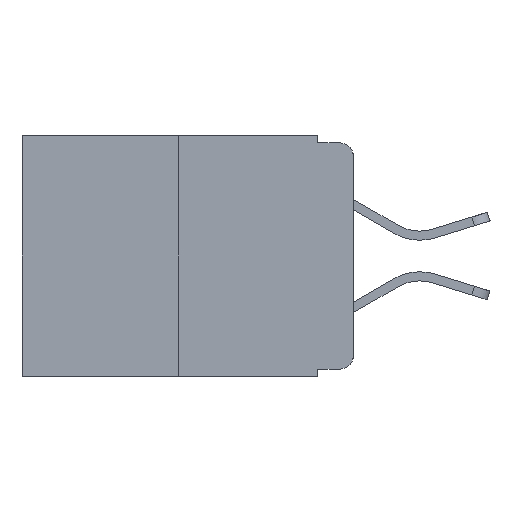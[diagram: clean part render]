
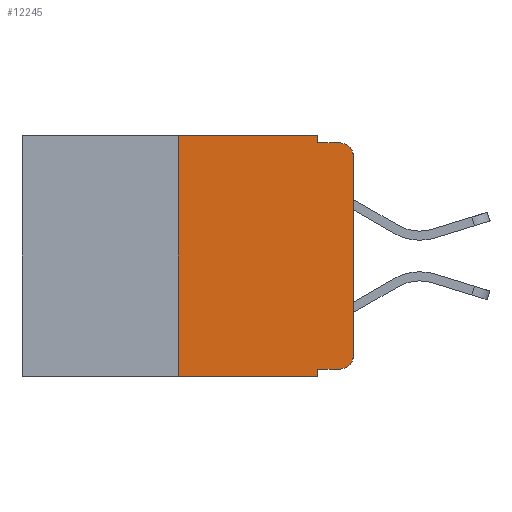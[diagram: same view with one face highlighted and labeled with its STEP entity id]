
A CAD part, left-side view. The second image highlights one B-rep face of the part: STEP entity #12245.
In plain terms, the highlighted planar face has unit normal (-1, 0, 0).
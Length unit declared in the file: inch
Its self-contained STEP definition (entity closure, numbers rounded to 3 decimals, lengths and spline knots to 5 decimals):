
#86 = VERTEX_POINT ( 'NONE', #8247 ) ;
#112 = AXIS2_PLACEMENT_3D ( 'NONE', #15344, #8192, #509 ) ;
#354 = VECTOR ( 'NONE', #6075, 39.37008 ) ;
#388 = AXIS2_PLACEMENT_3D ( 'NONE', #752, #9675, #2037 ) ;
#394 = VERTEX_POINT ( 'NONE', #9974 ) ;
#473 = VECTOR ( 'NONE', #12049, 39.37008 ) ;
#509 = DIRECTION ( 'NONE',  ( 0., 0., -1. ) ) ;
#511 = CARTESIAN_POINT ( 'NONE',  ( 0., 0.25, -0.343 ) ) ;
#539 = FACE_OUTER_BOUND ( 'NONE', #6815, .T. ) ;
#752 = CARTESIAN_POINT ( 'NONE',  ( 0., 0.02, -0.03 ) ) ;
#921 = ORIENTED_EDGE ( 'NONE', *, *, #13952, .F. ) ;
#991 = DIRECTION ( 'NONE',  ( 0., 0., -1. ) ) ;
#1040 = CARTESIAN_POINT ( 'NONE',  ( 0., 0.473, 0. ) ) ;
#1121 = EDGE_CURVE ( 'NONE', #3580, #394, #6750, .T. ) ;
#1469 = VECTOR ( 'NONE', #11101, 39.37008 ) ;
#2037 = DIRECTION ( 'NONE',  ( 0., 0., -1. ) ) ;
#2265 = CARTESIAN_POINT ( 'NONE',  ( 0., 0.051, -0.01 ) ) ;
#2468 = CARTESIAN_POINT ( 'NONE',  ( 0., 0.25, 0. ) ) ;
#2502 = CARTESIAN_POINT ( 'NONE',  ( 0., 0.051, -0.333 ) ) ;
#2577 = CARTESIAN_POINT ( 'NONE',  ( 0., 0.051, 0. ) ) ;
#2629 = VERTEX_POINT ( 'NONE', #511 ) ;
#2806 = EDGE_CURVE ( 'NONE', #86, #8967, #11943, .T. ) ;
#2962 = CARTESIAN_POINT ( 'NONE',  ( 0., 0.473, -0.343 ) ) ;
#3580 = VERTEX_POINT ( 'NONE', #2468 ) ;
#3797 = LINE ( 'NONE', #11043, #354 ) ;
#4529 = EDGE_CURVE ( 'NONE', #15846, #8967, #9618, .T. ) ;
#4538 = DIRECTION ( 'NONE',  ( 1., 0., 0. ) ) ;
#4542 = CARTESIAN_POINT ( 'NONE',  ( 0., 0.25, 0. ) ) ;
#5122 = LINE ( 'NONE', #4542, #473 ) ;
#5204 = VERTEX_POINT ( 'NONE', #5880 ) ;
#5337 = CARTESIAN_POINT ( 'NONE',  ( 0., 0., -0.03 ) ) ;
#5397 = EDGE_CURVE ( 'NONE', #5204, #15846, #10142, .T. ) ;
#5542 = CARTESIAN_POINT ( 'NONE',  ( 0., 0.051, -0.343 ) ) ;
#5880 = CARTESIAN_POINT ( 'NONE',  ( 0., 0., -0.313 ) ) ;
#6075 = DIRECTION ( 'NONE',  ( 0., -1., 0. ) ) ;
#6325 = CARTESIAN_POINT ( 'NONE',  ( 0., 0., 0. ) ) ;
#6484 = VECTOR ( 'NONE', #991, 39.37008 ) ;
#6600 = CARTESIAN_POINT ( 'NONE',  ( 0., 0.02, -0.01 ) ) ;
#6750 = LINE ( 'NONE', #1040, #7164 ) ;
#6815 = EDGE_LOOP ( 'NONE', ( #11377, #10442, #11582, #15055, #10259, #921, #8923, #11599, #9501, #13113 ) ) ;
#7164 = VECTOR ( 'NONE', #10302, 39.37008 ) ;
#7458 = CARTESIAN_POINT ( 'NONE',  ( 0., 0.02, -0.333 ) ) ;
#8192 = DIRECTION ( 'NONE',  ( -1., 0., 0. ) ) ;
#8247 = CARTESIAN_POINT ( 'NONE',  ( 0., 0.051, -0.01 ) ) ;
#8332 = CARTESIAN_POINT ( 'NONE',  ( 0., 0.473, 0. ) ) ;
#8361 = VECTOR ( 'NONE', #11383, 39.37008 ) ;
#8430 = VERTEX_POINT ( 'NONE', #5542 ) ;
#8923 = ORIENTED_EDGE ( 'NONE', *, *, #10052, .T. ) ;
#8967 = VERTEX_POINT ( 'NONE', #6600 ) ;
#9111 = EDGE_CURVE ( 'NONE', #11653, #5204, #13615, .T. ) ;
#9501 = ORIENTED_EDGE ( 'NONE', *, *, #11566, .T. ) ;
#9618 = CIRCLE ( 'NONE', #388, 0.02 ) ;
#9675 = DIRECTION ( 'NONE',  ( -1., 0., 0. ) ) ;
#9884 = CARTESIAN_POINT ( 'NONE',  ( 0., 0.051, 0. ) ) ;
#9974 = CARTESIAN_POINT ( 'NONE',  ( 0., 0.051, 0. ) ) ;
#10052 = EDGE_CURVE ( 'NONE', #2629, #8430, #15173, .T. ) ;
#10142 = LINE ( 'NONE', #6325, #10907 ) ;
#10209 = LINE ( 'NONE', #9884, #6484 ) ;
#10259 = ORIENTED_EDGE ( 'NONE', *, *, #1121, .F. ) ;
#10302 = DIRECTION ( 'NONE',  ( 0., -1., 0. ) ) ;
#10442 = ORIENTED_EDGE ( 'NONE', *, *, #4529, .T. ) ;
#10907 = VECTOR ( 'NONE', #14827, 39.37008 ) ;
#11043 = CARTESIAN_POINT ( 'NONE',  ( 0., 0.051, -0.333 ) ) ;
#11101 = DIRECTION ( 'NONE',  ( 0., -1., 0. ) ) ;
#11377 = ORIENTED_EDGE ( 'NONE', *, *, #5397, .T. ) ;
#11383 = DIRECTION ( 'NONE',  ( 0., 0., -1. ) ) ;
#11566 = EDGE_CURVE ( 'NONE', #15143, #11653, #3797, .T. ) ;
#11582 = ORIENTED_EDGE ( 'NONE', *, *, #2806, .F. ) ;
#11599 = ORIENTED_EDGE ( 'NONE', *, *, #12405, .F. ) ;
#11653 = VERTEX_POINT ( 'NONE', #7458 ) ;
#11780 = DIRECTION ( 'NONE',  ( 0., -1., 0. ) ) ;
#11943 = LINE ( 'NONE', #2265, #1469 ) ;
#12049 = DIRECTION ( 'NONE',  ( 0., 0., 1. ) ) ;
#12116 = VECTOR ( 'NONE', #11780, 39.37008 ) ;
#12245 = ADVANCED_FACE ( 'NONE', ( #539 ), #15472, .F. ) ;
#12405 = EDGE_CURVE ( 'NONE', #15143, #8430, #14033, .T. ) ;
#13113 = ORIENTED_EDGE ( 'NONE', *, *, #9111, .T. ) ;
#13245 = DIRECTION ( 'NONE',  ( 0., 0., -1. ) ) ;
#13615 = CIRCLE ( 'NONE', #112, 0.02 ) ;
#13952 = EDGE_CURVE ( 'NONE', #2629, #3580, #5122, .T. ) ;
#14033 = LINE ( 'NONE', #2577, #8361 ) ;
#14723 = EDGE_CURVE ( 'NONE', #394, #86, #10209, .T. ) ;
#14827 = DIRECTION ( 'NONE',  ( 0., 0., 1. ) ) ;
#15055 = ORIENTED_EDGE ( 'NONE', *, *, #14723, .F. ) ;
#15143 = VERTEX_POINT ( 'NONE', #2502 ) ;
#15150 = AXIS2_PLACEMENT_3D ( 'NONE', #8332, #4538, #13245 ) ;
#15173 = LINE ( 'NONE', #2962, #12116 ) ;
#15344 = CARTESIAN_POINT ( 'NONE',  ( 0., 0.02, -0.313 ) ) ;
#15472 = PLANE ( 'NONE',  #15150 ) ;
#15846 = VERTEX_POINT ( 'NONE', #5337 ) ;
